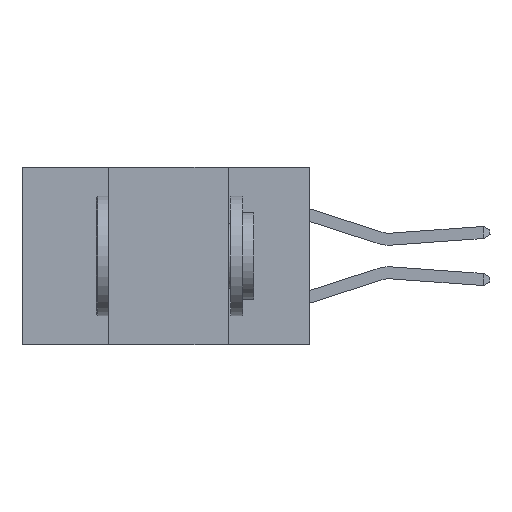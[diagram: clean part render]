
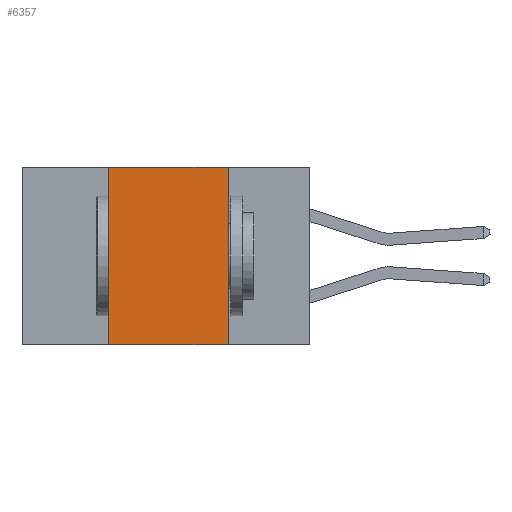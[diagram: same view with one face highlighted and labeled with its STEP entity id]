
A CAD part, left-side view. The second image highlights one B-rep face of the part: STEP entity #6357.
In plain terms, the highlighted planar face has unit normal (-1, 0, 0).
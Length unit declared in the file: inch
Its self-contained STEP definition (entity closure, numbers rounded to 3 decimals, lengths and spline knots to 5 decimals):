
#310 = EDGE_CURVE ( 'NONE', #572, #7989, #9349, .T. ) ;
#382 = ORIENTED_EDGE ( 'NONE', *, *, #670, .F. ) ;
#572 = VERTEX_POINT ( 'NONE', #6095 ) ;
#670 = EDGE_CURVE ( 'NONE', #4171, #572, #8271, .T. ) ;
#1453 = VECTOR ( 'NONE', #1758, 39.37008 ) ;
#1469 = ORIENTED_EDGE ( 'NONE', *, *, #2695, .F. ) ;
#1758 = DIRECTION ( 'NONE',  ( 0., 0., 1. ) ) ;
#1825 = LINE ( 'NONE', #5668, #7427 ) ;
#2456 = EDGE_CURVE ( 'NONE', #4171, #3165, #1825, .T. ) ;
#2671 = DIRECTION ( 'NONE',  ( 0., -1., 0. ) ) ;
#2695 = EDGE_CURVE ( 'NONE', #7989, #3165, #4615, .T. ) ;
#3119 = ORIENTED_EDGE ( 'NONE', *, *, #2456, .T. ) ;
#3132 = CARTESIAN_POINT ( 'NONE',  ( 0., 0.42, -0.37 ) ) ;
#3158 = DIRECTION ( 'NONE',  ( 0., 0., -1. ) ) ;
#3165 = VERTEX_POINT ( 'NONE', #4510 ) ;
#3342 = PLANE ( 'NONE',  #4748 ) ;
#3800 = VECTOR ( 'NONE', #8891, 39.37008 ) ;
#4171 = VERTEX_POINT ( 'NONE', #4948 ) ;
#4203 = EDGE_LOOP ( 'NONE', ( #1469, #9171, #382, #3119 ) ) ;
#4510 = CARTESIAN_POINT ( 'NONE',  ( 0., 0.17, -0.37 ) ) ;
#4615 = LINE ( 'NONE', #6004, #3800 ) ;
#4748 = AXIS2_PLACEMENT_3D ( 'NONE', #7691, #7542, #3158 ) ;
#4786 = FACE_OUTER_BOUND ( 'NONE', #4203, .T. ) ;
#4948 = CARTESIAN_POINT ( 'NONE',  ( 0., 0.42, -0.37 ) ) ;
#5570 = CARTESIAN_POINT ( 'NONE',  ( 0., 0.6, 0. ) ) ;
#5668 = CARTESIAN_POINT ( 'NONE',  ( 0., 0.6, -0.37 ) ) ;
#6004 = CARTESIAN_POINT ( 'NONE',  ( 0., 0.17, -0.37 ) ) ;
#6095 = CARTESIAN_POINT ( 'NONE',  ( 0., 0.42, 0. ) ) ;
#6357 = ADVANCED_FACE ( 'NONE', ( #4786 ), #3342, .F. ) ;
#6632 = VECTOR ( 'NONE', #8598, 39.37008 ) ;
#7427 = VECTOR ( 'NONE', #2671, 39.37008 ) ;
#7542 = DIRECTION ( 'NONE',  ( 1., 0., 0. ) ) ;
#7691 = CARTESIAN_POINT ( 'NONE',  ( 0., 0.6, 0. ) ) ;
#7904 = CARTESIAN_POINT ( 'NONE',  ( 0., 0.17, 0. ) ) ;
#7989 = VERTEX_POINT ( 'NONE', #7904 ) ;
#8271 = LINE ( 'NONE', #3132, #1453 ) ;
#8598 = DIRECTION ( 'NONE',  ( 0., -1., 0. ) ) ;
#8891 = DIRECTION ( 'NONE',  ( 0., 0., -1. ) ) ;
#9171 = ORIENTED_EDGE ( 'NONE', *, *, #310, .F. ) ;
#9349 = LINE ( 'NONE', #5570, #6632 ) ;
